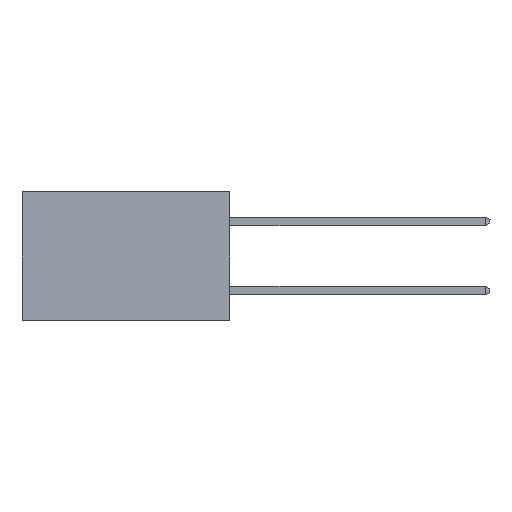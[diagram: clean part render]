
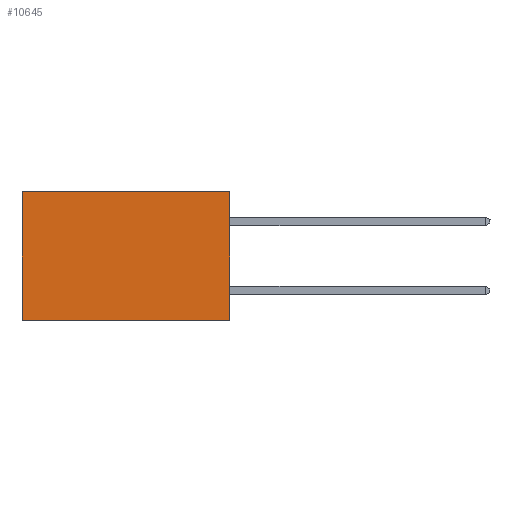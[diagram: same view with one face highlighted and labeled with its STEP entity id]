
A CAD part, left-side view. The second image highlights one B-rep face of the part: STEP entity #10645.
In plain terms, the highlighted planar face has unit normal (-1, 0, 0).
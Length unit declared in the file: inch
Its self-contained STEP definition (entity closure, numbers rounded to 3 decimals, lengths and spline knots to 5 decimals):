
#478 = VECTOR ( 'NONE', #15109, 39.37008 ) ;
#683 = ORIENTED_EDGE ( 'NONE', *, *, #6099, .F. ) ;
#1315 = EDGE_CURVE ( 'NONE', #9806, #11594, #3054, .T. ) ;
#1962 = LINE ( 'NONE', #9923, #9102 ) ;
#2059 = DIRECTION ( 'NONE',  ( 0., 0., -1. ) ) ;
#2845 = CARTESIAN_POINT ( 'NONE',  ( 0.2615, 0.6, 0. ) ) ;
#3054 = LINE ( 'NONE', #8203, #8997 ) ;
#3808 = CARTESIAN_POINT ( 'NONE',  ( 0.2615, 0., -0.37 ) ) ;
#4720 = CARTESIAN_POINT ( 'NONE',  ( 0.2615, 0., -0.37 ) ) ;
#5074 = FACE_OUTER_BOUND ( 'NONE', #7914, .T. ) ;
#6099 = EDGE_CURVE ( 'NONE', #11518, #9806, #1962, .T. ) ;
#7542 = AXIS2_PLACEMENT_3D ( 'NONE', #3808, #8963, #7855 ) ;
#7614 = LINE ( 'NONE', #15352, #478 ) ;
#7855 = DIRECTION ( 'NONE',  ( 0., 0., -1. ) ) ;
#7914 = EDGE_LOOP ( 'NONE', ( #14919, #16714, #683, #10204 ) ) ;
#8203 = CARTESIAN_POINT ( 'NONE',  ( 0.2615, 0., -0.37 ) ) ;
#8963 = DIRECTION ( 'NONE',  ( 1., 0., 0. ) ) ;
#8997 = VECTOR ( 'NONE', #12121, 39.37008 ) ;
#9102 = VECTOR ( 'NONE', #13683, 39.37008 ) ;
#9176 = EDGE_CURVE ( 'NONE', #13334, #11594, #9681, .T. ) ;
#9681 = LINE ( 'NONE', #14892, #16201 ) ;
#9806 = VERTEX_POINT ( 'NONE', #4720 ) ;
#9923 = CARTESIAN_POINT ( 'NONE',  ( 0.2615, 0., -0.37 ) ) ;
#10204 = ORIENTED_EDGE ( 'NONE', *, *, #10635, .T. ) ;
#10247 = PLANE ( 'NONE',  #7542 ) ;
#10635 = EDGE_CURVE ( 'NONE', #11518, #13334, #7614, .T. ) ;
#10645 = ADVANCED_FACE ( 'NONE', ( #5074 ), #10247, .F. ) ;
#10750 = CARTESIAN_POINT ( 'NONE',  ( 0.2615, 0.6, -0.37 ) ) ;
#11518 = VERTEX_POINT ( 'NONE', #11857 ) ;
#11594 = VERTEX_POINT ( 'NONE', #10750 ) ;
#11857 = CARTESIAN_POINT ( 'NONE',  ( 0.2615, 0., 0. ) ) ;
#12121 = DIRECTION ( 'NONE',  ( 0., 1., 0. ) ) ;
#13334 = VERTEX_POINT ( 'NONE', #2845 ) ;
#13683 = DIRECTION ( 'NONE',  ( 0., 0., -1. ) ) ;
#14892 = CARTESIAN_POINT ( 'NONE',  ( 0.2615, 0.6, -0.37 ) ) ;
#14919 = ORIENTED_EDGE ( 'NONE', *, *, #9176, .T. ) ;
#15109 = DIRECTION ( 'NONE',  ( 0., 1., 0. ) ) ;
#15352 = CARTESIAN_POINT ( 'NONE',  ( 0.2615, 0., 0. ) ) ;
#16201 = VECTOR ( 'NONE', #2059, 39.37008 ) ;
#16714 = ORIENTED_EDGE ( 'NONE', *, *, #1315, .F. ) ;
